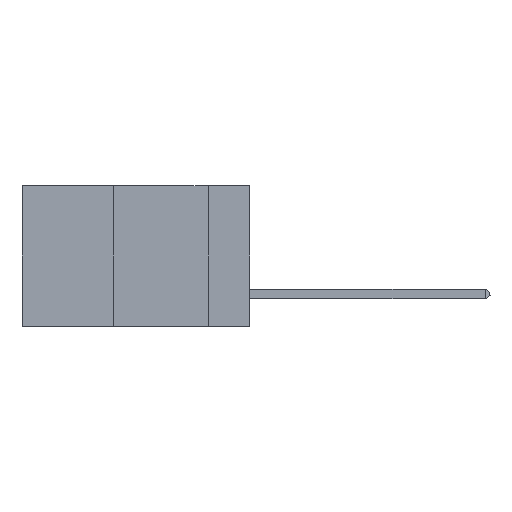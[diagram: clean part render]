
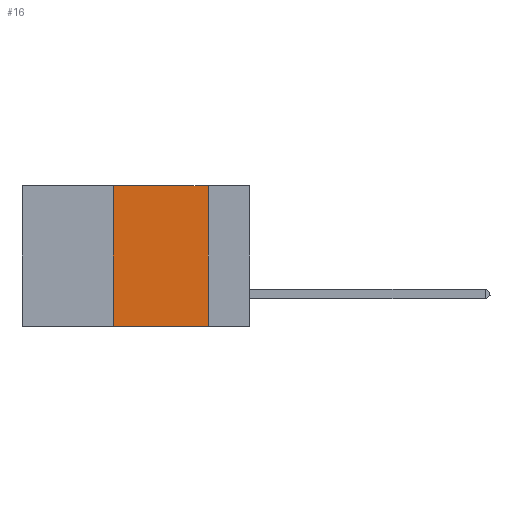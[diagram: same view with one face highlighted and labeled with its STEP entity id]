
A CAD part, left-side view. The second image highlights one B-rep face of the part: STEP entity #16.
In plain terms, the highlighted planar face has unit normal (-1, 0, 0).
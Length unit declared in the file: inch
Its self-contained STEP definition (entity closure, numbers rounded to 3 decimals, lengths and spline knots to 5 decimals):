
#16 = ADVANCED_FACE ( 'NONE', ( #12480 ), #5875, .F. ) ;
#61 = EDGE_CURVE ( 'NONE', #20588, #20825, #8736, .T. ) ;
#1035 = DIRECTION ( 'NONE',  ( 0., -1., 0. ) ) ;
#3730 = DIRECTION ( 'NONE',  ( 1., 0., 0. ) ) ;
#3748 = CARTESIAN_POINT ( 'NONE',  ( 0., 0.36, -0.37 ) ) ;
#5875 = PLANE ( 'NONE',  #6204 ) ;
#6204 = AXIS2_PLACEMENT_3D ( 'NONE', #15167, #3730, #19706 ) ;
#8736 = LINE ( 'NONE', #13572, #28488 ) ;
#10326 = CARTESIAN_POINT ( 'NONE',  ( 0., 0.6, -0.37 ) ) ;
#10663 = CARTESIAN_POINT ( 'NONE',  ( 0., 0.6, 0. ) ) ;
#11150 = CARTESIAN_POINT ( 'NONE',  ( 0., 0.36, 0. ) ) ;
#11416 = VECTOR ( 'NONE', #17173, 39.37008 ) ;
#12480 = FACE_OUTER_BOUND ( 'NONE', #13652, .T. ) ;
#12630 = VECTOR ( 'NONE', #27006, 39.37008 ) ;
#12953 = EDGE_CURVE ( 'NONE', #20588, #19476, #18964, .T. ) ;
#13559 = ORIENTED_EDGE ( 'NONE', *, *, #18318, .F. ) ;
#13572 = CARTESIAN_POINT ( 'NONE',  ( 0., 0.36, 0. ) ) ;
#13652 = EDGE_LOOP ( 'NONE', ( #29508, #13559, #26013, #16621 ) ) ;
#14338 = CARTESIAN_POINT ( 'NONE',  ( 0., 0.11, -0.37 ) ) ;
#15167 = CARTESIAN_POINT ( 'NONE',  ( 0., 0.6, 0. ) ) ;
#15529 = EDGE_CURVE ( 'NONE', #21509, #19476, #18398, .T. ) ;
#16621 = ORIENTED_EDGE ( 'NONE', *, *, #12953, .T. ) ;
#17173 = DIRECTION ( 'NONE',  ( 0., -1., 0. ) ) ;
#18318 = EDGE_CURVE ( 'NONE', #20825, #21509, #20715, .T. ) ;
#18398 = LINE ( 'NONE', #24692, #12630 ) ;
#18964 = LINE ( 'NONE', #10326, #11416 ) ;
#19476 = VERTEX_POINT ( 'NONE', #14338 ) ;
#19706 = DIRECTION ( 'NONE',  ( 0., 0., -1. ) ) ;
#20588 = VERTEX_POINT ( 'NONE', #3748 ) ;
#20715 = LINE ( 'NONE', #10663, #28215 ) ;
#20825 = VERTEX_POINT ( 'NONE', #11150 ) ;
#21509 = VERTEX_POINT ( 'NONE', #25257 ) ;
#24692 = CARTESIAN_POINT ( 'NONE',  ( 0., 0.11, 0. ) ) ;
#25257 = CARTESIAN_POINT ( 'NONE',  ( 0., 0.11, 0. ) ) ;
#26013 = ORIENTED_EDGE ( 'NONE', *, *, #61, .F. ) ;
#27006 = DIRECTION ( 'NONE',  ( 0., 0., -1. ) ) ;
#27417 = DIRECTION ( 'NONE',  ( 0., 0., 1. ) ) ;
#28215 = VECTOR ( 'NONE', #1035, 39.37008 ) ;
#28488 = VECTOR ( 'NONE', #27417, 39.37008 ) ;
#29508 = ORIENTED_EDGE ( 'NONE', *, *, #15529, .F. ) ;
